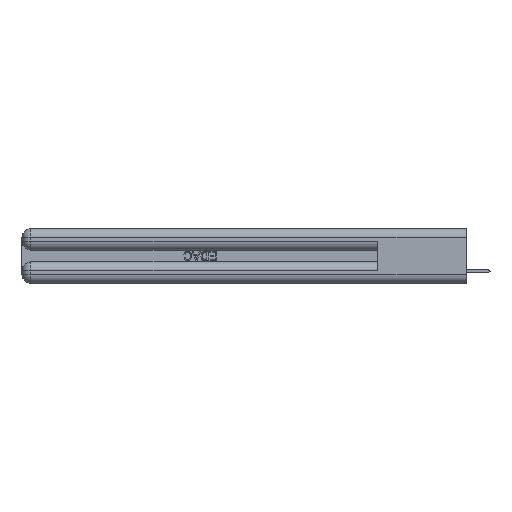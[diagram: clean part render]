
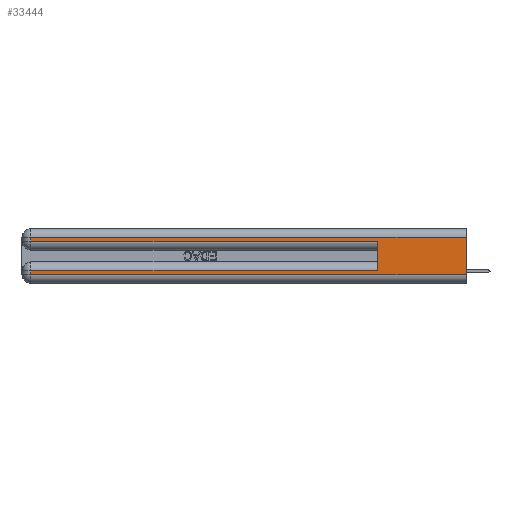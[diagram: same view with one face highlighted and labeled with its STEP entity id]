
A CAD part, left-side view. The second image highlights one B-rep face of the part: STEP entity #33444.
In plain terms, the highlighted planar face has unit normal (-1, 0, 0).
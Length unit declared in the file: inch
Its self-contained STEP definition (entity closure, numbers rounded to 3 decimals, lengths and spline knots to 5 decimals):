
#218 = FACE_OUTER_BOUND ( 'NONE', #33279, .T. ) ;
#2273 = VECTOR ( 'NONE', #45151, 39.37008 ) ;
#2420 = EDGE_CURVE ( 'NONE', #13127, #16860, #36987, .T. ) ;
#3259 = ORIENTED_EDGE ( 'NONE', *, *, #29153, .T. ) ;
#4901 = CARTESIAN_POINT ( 'NONE',  ( 0., 2.94, 0.285 ) ) ;
#4907 = EDGE_CURVE ( 'NONE', #20297, #40109, #20001, .T. ) ;
#4928 = EDGE_CURVE ( 'NONE', #16860, #16978, #46078, .T. ) ;
#5216 = CARTESIAN_POINT ( 'NONE',  ( 0., 0., 0.37 ) ) ;
#5323 = DIRECTION ( 'NONE',  ( 0., 1., 0. ) ) ;
#5371 = DIRECTION ( 'NONE',  ( 0., 0., -1. ) ) ;
#5758 = VERTEX_POINT ( 'NONE', #12472 ) ;
#6126 = LINE ( 'NONE', #34144, #6684 ) ;
#6501 = EDGE_CURVE ( 'NONE', #20297, #13127, #33160, .T. ) ;
#6684 = VECTOR ( 'NONE', #33660, 39.37008 ) ;
#8648 = VECTOR ( 'NONE', #34592, 39.37008 ) ;
#8732 = CARTESIAN_POINT ( 'NONE',  ( 0., 2.94, 0.37 ) ) ;
#9109 = DIRECTION ( 'NONE',  ( 0., 1., 0. ) ) ;
#9630 = VECTOR ( 'NONE', #34373, 39.37008 ) ;
#11356 = VECTOR ( 'NONE', #38886, 39.37008 ) ;
#12472 = CARTESIAN_POINT ( 'NONE',  ( 0., 0., 0.31 ) ) ;
#13127 = VERTEX_POINT ( 'NONE', #37305 ) ;
#13833 = ORIENTED_EDGE ( 'NONE', *, *, #4907, .F. ) ;
#13915 = CARTESIAN_POINT ( 'NONE',  ( 0., 0., 0.06 ) ) ;
#14411 = DIRECTION ( 'NONE',  ( 1., 0., 0. ) ) ;
#16860 = VERTEX_POINT ( 'NONE', #47172 ) ;
#16978 = VERTEX_POINT ( 'NONE', #13915 ) ;
#18139 = VECTOR ( 'NONE', #9109, 39.37008 ) ;
#19089 = ORIENTED_EDGE ( 'NONE', *, *, #6501, .T. ) ;
#19278 = LINE ( 'NONE', #42271, #18139 ) ;
#19688 = CARTESIAN_POINT ( 'NONE',  ( 0., 0., 0.085 ) ) ;
#20000 = ORIENTED_EDGE ( 'NONE', *, *, #4928, .T. ) ;
#20001 = LINE ( 'NONE', #45541, #9630 ) ;
#20297 = VERTEX_POINT ( 'NONE', #25983 ) ;
#20467 = VERTEX_POINT ( 'NONE', #4901 ) ;
#21136 = LINE ( 'NONE', #5216, #22866 ) ;
#21650 = DIRECTION ( 'NONE',  ( 0., 0., -1. ) ) ;
#22317 = CARTESIAN_POINT ( 'NONE',  ( 0., 0.6, 0.285 ) ) ;
#22866 = VECTOR ( 'NONE', #5371, 39.37008 ) ;
#23154 = AXIS2_PLACEMENT_3D ( 'NONE', #40130, #14411, #21650 ) ;
#23564 = ORIENTED_EDGE ( 'NONE', *, *, #31783, .T. ) ;
#25983 = CARTESIAN_POINT ( 'NONE',  ( 0., 0.6, 0.085 ) ) ;
#27337 = ORIENTED_EDGE ( 'NONE', *, *, #46110, .F. ) ;
#27773 = EDGE_CURVE ( 'NONE', #20467, #40109, #6126, .T. ) ;
#29153 = EDGE_CURVE ( 'NONE', #5758, #36106, #19278, .T. ) ;
#29942 = ORIENTED_EDGE ( 'NONE', *, *, #27773, .T. ) ;
#30593 = LINE ( 'NONE', #33824, #2273 ) ;
#31406 = VECTOR ( 'NONE', #5323, 39.37008 ) ;
#31783 = EDGE_CURVE ( 'NONE', #36106, #20467, #30593, .T. ) ;
#33160 = LINE ( 'NONE', #19688, #31406 ) ;
#33279 = EDGE_LOOP ( 'NONE', ( #27337, #3259, #23564, #29942, #13833, #19089, #42904, #20000 ) ) ;
#33391 = CARTESIAN_POINT ( 'NONE',  ( 0., 2.94, 0.31 ) ) ;
#33444 = ADVANCED_FACE ( 'NONE', ( #218 ), #36385, .F. ) ;
#33660 = DIRECTION ( 'NONE',  ( 0., -1., 0. ) ) ;
#33824 = CARTESIAN_POINT ( 'NONE',  ( 0., 2.94, 0.37 ) ) ;
#34144 = CARTESIAN_POINT ( 'NONE',  ( 0., 0., 0.285 ) ) ;
#34373 = DIRECTION ( 'NONE',  ( 0., 0., 1. ) ) ;
#34592 = DIRECTION ( 'NONE',  ( 0., 0., -1. ) ) ;
#36106 = VERTEX_POINT ( 'NONE', #33391 ) ;
#36385 = PLANE ( 'NONE',  #23154 ) ;
#36987 = LINE ( 'NONE', #8732, #8648 ) ;
#37305 = CARTESIAN_POINT ( 'NONE',  ( 0., 2.94, 0.085 ) ) ;
#38886 = DIRECTION ( 'NONE',  ( 0., -1., 0. ) ) ;
#40109 = VERTEX_POINT ( 'NONE', #22317 ) ;
#40130 = CARTESIAN_POINT ( 'NONE',  ( 0., 0., 0.37 ) ) ;
#42271 = CARTESIAN_POINT ( 'NONE',  ( 0., 0., 0.31 ) ) ;
#42904 = ORIENTED_EDGE ( 'NONE', *, *, #2420, .T. ) ;
#45151 = DIRECTION ( 'NONE',  ( 0., 0., -1. ) ) ;
#45541 = CARTESIAN_POINT ( 'NONE',  ( 0., 0.6, 0.145 ) ) ;
#45700 = CARTESIAN_POINT ( 'NONE',  ( 0., 0., 0.06 ) ) ;
#46078 = LINE ( 'NONE', #45700, #11356 ) ;
#46110 = EDGE_CURVE ( 'NONE', #5758, #16978, #21136, .T. ) ;
#47172 = CARTESIAN_POINT ( 'NONE',  ( 0., 2.94, 0.06 ) ) ;
